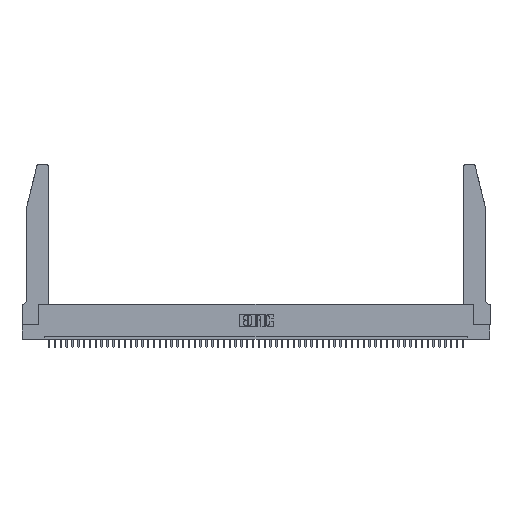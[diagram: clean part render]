
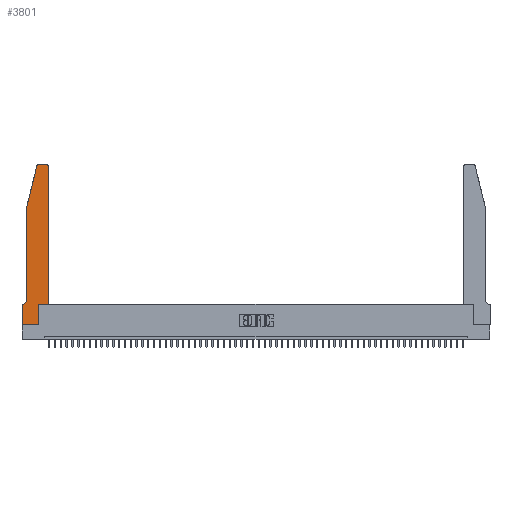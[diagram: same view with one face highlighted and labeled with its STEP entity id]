
A CAD part, top view. The second image highlights one B-rep face of the part: STEP entity #3801.
In plain terms, the highlighted planar face has unit normal (0, 0, 1).
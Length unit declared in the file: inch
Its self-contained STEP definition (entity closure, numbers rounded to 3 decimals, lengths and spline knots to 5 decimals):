
#1386 = LINE ( 'NONE', #30552, #10002 ) ;
#2700 = VERTEX_POINT ( 'NONE', #30526 ) ;
#3244 = ORIENTED_EDGE ( 'NONE', *, *, #34287, .T. ) ;
#3294 = LINE ( 'NONE', #9647, #14581 ) ;
#3745 = VERTEX_POINT ( 'NONE', #17103 ) ;
#3801 = ADVANCED_FACE ( 'NONE', ( #9775 ), #16732, .T. ) ;
#4295 = DIRECTION ( 'NONE',  ( 0., 0., 1. ) ) ;
#5237 = VECTOR ( 'NONE', #5337, 39.37008 ) ;
#5256 = EDGE_CURVE ( 'NONE', #3745, #51161, #6896, .T. ) ;
#5337 = DIRECTION ( 'NONE',  ( -1., 0., 0. ) ) ;
#5404 = CARTESIAN_POINT ( 'NONE',  ( 0.0055, 0.42, 0.37 ) ) ;
#5524 = VERTEX_POINT ( 'NONE', #34005 ) ;
#5532 = ORIENTED_EDGE ( 'NONE', *, *, #6341, .T. ) ;
#6023 = ORIENTED_EDGE ( 'NONE', *, *, #5256, .T. ) ;
#6341 = EDGE_CURVE ( 'NONE', #29663, #31510, #51920, .T. ) ;
#6896 = LINE ( 'NONE', #52302, #8197 ) ;
#7082 = CARTESIAN_POINT ( 'NONE',  ( 0.4505, 2.72, 0.37 ) ) ;
#7561 = EDGE_LOOP ( 'NONE', ( #24688, #14440, #15656, #8671, #5532, #52996, #8313, #21870, #28787, #6023, #3244, #43777 ) ) ;
#7786 = EDGE_CURVE ( 'NONE', #31510, #45637, #43398, .T. ) ;
#7787 = CIRCLE ( 'NONE', #52577, 0.03 ) ;
#8197 = VECTOR ( 'NONE', #9510, 39.37008 ) ;
#8313 = ORIENTED_EDGE ( 'NONE', *, *, #34537, .T. ) ;
#8347 = CARTESIAN_POINT ( 'NONE',  ( 0.0755, 2., 0.37 ) ) ;
#8671 = ORIENTED_EDGE ( 'NONE', *, *, #27572, .T. ) ;
#9388 = CARTESIAN_POINT ( 'NONE',  ( 0.284, 2.72, 0.37 ) ) ;
#9510 = DIRECTION ( 'NONE',  ( 1., 0., 0. ) ) ;
#9647 = CARTESIAN_POINT ( 'NONE',  ( 0.0755, 2., 0.37 ) ) ;
#9775 = FACE_OUTER_BOUND ( 'NONE', #7561, .T. ) ;
#10002 = VECTOR ( 'NONE', #34399, 39.37008 ) ;
#10226 = CARTESIAN_POINT ( 'NONE',  ( 0.4505, 0.35, 0.37 ) ) ;
#10883 = EDGE_CURVE ( 'NONE', #5524, #47821, #13252, .T. ) ;
#11684 = VECTOR ( 'NONE', #47639, 39.37008 ) ;
#11918 = CARTESIAN_POINT ( 'NONE',  ( 0.2605, 2.75, 0.37 ) ) ;
#13252 = LINE ( 'NONE', #11918, #5237 ) ;
#13881 = DIRECTION ( 'NONE',  ( 1., 0., 0. ) ) ;
#14161 = DIRECTION ( 'NONE',  ( -1., 0., 0. ) ) ;
#14440 = ORIENTED_EDGE ( 'NONE', *, *, #54142, .T. ) ;
#14581 = VECTOR ( 'NONE', #26334, 39.37008 ) ;
#14729 = VERTEX_POINT ( 'NONE', #50672 ) ;
#15656 = ORIENTED_EDGE ( 'NONE', *, *, #53346, .T. ) ;
#15663 = VECTOR ( 'NONE', #27964, 39.37008 ) ;
#16732 = PLANE ( 'NONE',  #22693 ) ;
#16915 = DIRECTION ( 'NONE',  ( -0.239, -0.971, 0. ) ) ;
#17103 = CARTESIAN_POINT ( 'NONE',  ( 0.2865, 0.35, 0.37 ) ) ;
#17270 = CARTESIAN_POINT ( 'NONE',  ( 0., 0.35, 0.37 ) ) ;
#17453 = DIRECTION ( 'NONE',  ( 1., 0., 0. ) ) ;
#19616 = CARTESIAN_POINT ( 'NONE',  ( 0.0755, 0.42, 0.37 ) ) ;
#19688 = DIRECTION ( 'NONE',  ( 1., 0., 0. ) ) ;
#21150 = EDGE_CURVE ( 'NONE', #2700, #3745, #29756, .T. ) ;
#21527 = EDGE_CURVE ( 'NONE', #25091, #5524, #27742, .T. ) ;
#21870 = ORIENTED_EDGE ( 'NONE', *, *, #45691, .T. ) ;
#22693 = AXIS2_PLACEMENT_3D ( 'NONE', #17270, #4295, #17453 ) ;
#22776 = AXIS2_PLACEMENT_3D ( 'NONE', #5404, #22851, #14161 ) ;
#22851 = DIRECTION ( 'NONE',  ( 0., 0., -1. ) ) ;
#24688 = ORIENTED_EDGE ( 'NONE', *, *, #10883, .T. ) ;
#25091 = VERTEX_POINT ( 'NONE', #7082 ) ;
#26334 = DIRECTION ( 'NONE',  ( 0., -1., 0. ) ) ;
#26914 = LINE ( 'NONE', #53011, #15663 ) ;
#27470 = CARTESIAN_POINT ( 'NONE',  ( 0.25487, 2.72718, 0.37 ) ) ;
#27572 = EDGE_CURVE ( 'NONE', #14729, #29663, #3294, .T. ) ;
#27742 = CIRCLE ( 'NONE', #29250, 0.03 ) ;
#27964 = DIRECTION ( 'NONE',  ( 0., -1., 0. ) ) ;
#28761 = CARTESIAN_POINT ( 'NONE',  ( 0., 0., 0.37 ) ) ;
#28787 = ORIENTED_EDGE ( 'NONE', *, *, #21150, .T. ) ;
#29169 = CARTESIAN_POINT ( 'NONE',  ( 0.0755, 0.35, 0.37 ) ) ;
#29250 = AXIS2_PLACEMENT_3D ( 'NONE', #36155, #44861, #19688 ) ;
#29663 = VERTEX_POINT ( 'NONE', #19616 ) ;
#29756 = LINE ( 'NONE', #50256, #53657 ) ;
#30526 = CARTESIAN_POINT ( 'NONE',  ( 0.2865, 0., 0.37 ) ) ;
#30537 = DIRECTION ( 'NONE',  ( 0., 0., 1. ) ) ;
#30552 = CARTESIAN_POINT ( 'NONE',  ( 0., 0., 0.37 ) ) ;
#31510 = VERTEX_POINT ( 'NONE', #53325 ) ;
#34005 = CARTESIAN_POINT ( 'NONE',  ( 0.4205, 2.75, 0.37 ) ) ;
#34287 = EDGE_CURVE ( 'NONE', #51161, #25091, #54097, .T. ) ;
#34399 = DIRECTION ( 'NONE',  ( 1., 0., 0. ) ) ;
#34537 = EDGE_CURVE ( 'NONE', #45637, #49706, #26914, .T. ) ;
#36155 = CARTESIAN_POINT ( 'NONE',  ( 0.4205, 2.72, 0.37 ) ) ;
#36242 = CARTESIAN_POINT ( 'NONE',  ( 0.284, 2.75, 0.37 ) ) ;
#38671 = CARTESIAN_POINT ( 'NONE',  ( 0., 0.35, 0.37 ) ) ;
#39090 = CARTESIAN_POINT ( 'NONE',  ( 0.4505, 0.35, 0.37 ) ) ;
#39414 = VECTOR ( 'NONE', #46221, 39.37008 ) ;
#40795 = VERTEX_POINT ( 'NONE', #27470 ) ;
#43398 = LINE ( 'NONE', #29169, #39414 ) ;
#43777 = ORIENTED_EDGE ( 'NONE', *, *, #21527, .T. ) ;
#44861 = DIRECTION ( 'NONE',  ( 0., 0., 1. ) ) ;
#45637 = VERTEX_POINT ( 'NONE', #38671 ) ;
#45691 = EDGE_CURVE ( 'NONE', #49706, #2700, #1386, .T. ) ;
#46221 = DIRECTION ( 'NONE',  ( -1., 0., 0. ) ) ;
#46283 = VECTOR ( 'NONE', #16915, 39.37008 ) ;
#47639 = DIRECTION ( 'NONE',  ( 0., 1., 0. ) ) ;
#47821 = VERTEX_POINT ( 'NONE', #36242 ) ;
#48972 = LINE ( 'NONE', #8347, #46283 ) ;
#49706 = VERTEX_POINT ( 'NONE', #28761 ) ;
#50256 = CARTESIAN_POINT ( 'NONE',  ( 0.2865, 0.35, 0.37 ) ) ;
#50672 = CARTESIAN_POINT ( 'NONE',  ( 0.0755, 2., 0.37 ) ) ;
#51161 = VERTEX_POINT ( 'NONE', #10226 ) ;
#51920 = CIRCLE ( 'NONE', #22776, 0.07 ) ;
#52302 = CARTESIAN_POINT ( 'NONE',  ( 0.4505, 0.35, 0.37 ) ) ;
#52577 = AXIS2_PLACEMENT_3D ( 'NONE', #9388, #30537, #13881 ) ;
#52996 = ORIENTED_EDGE ( 'NONE', *, *, #7786, .T. ) ;
#53011 = CARTESIAN_POINT ( 'NONE',  ( 0., 0., 0.37 ) ) ;
#53325 = CARTESIAN_POINT ( 'NONE',  ( 0.0055, 0.35, 0.37 ) ) ;
#53346 = EDGE_CURVE ( 'NONE', #40795, #14729, #48972, .T. ) ;
#53657 = VECTOR ( 'NONE', #54726, 39.37008 ) ;
#54097 = LINE ( 'NONE', #39090, #11684 ) ;
#54142 = EDGE_CURVE ( 'NONE', #47821, #40795, #7787, .T. ) ;
#54726 = DIRECTION ( 'NONE',  ( 0., 1., 0. ) ) ;
